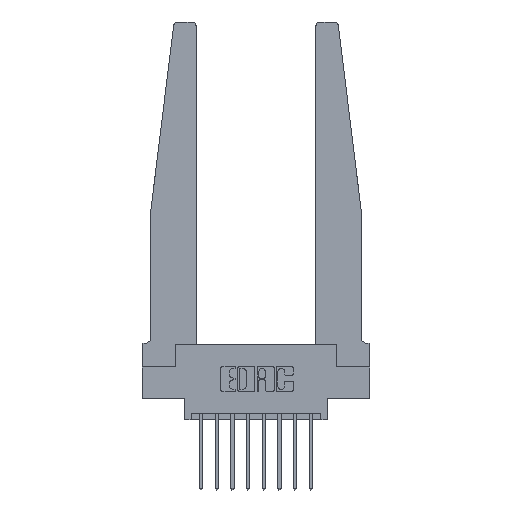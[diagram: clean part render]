
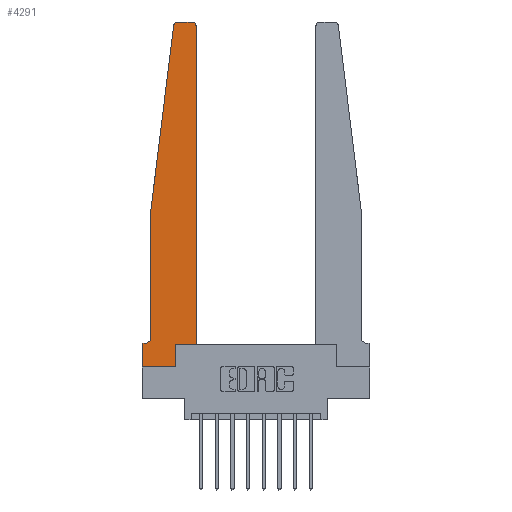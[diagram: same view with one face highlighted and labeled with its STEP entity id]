
A CAD part, top view. The second image highlights one B-rep face of the part: STEP entity #4291.
In plain terms, the highlighted planar face has unit normal (0, 0, 1).
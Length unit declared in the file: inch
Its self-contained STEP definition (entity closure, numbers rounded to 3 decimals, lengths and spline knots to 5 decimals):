
#67 = EDGE_CURVE ( 'NONE', #9984, #3799, #6321, .T. ) ;
#193 = VECTOR ( 'NONE', #11996, 39.37008 ) ;
#274 = EDGE_CURVE ( 'NONE', #8454, #6829, #14087, .T. ) ;
#299 = ORIENTED_EDGE ( 'NONE', *, *, #14269, .T. ) ;
#716 = EDGE_CURVE ( 'NONE', #3799, #8982, #1531, .T. ) ;
#754 = ORIENTED_EDGE ( 'NONE', *, *, #9614, .T. ) ;
#1057 = DIRECTION ( 'NONE',  ( -1., 0., 0. ) ) ;
#1059 = EDGE_CURVE ( 'NONE', #12440, #3065, #4650, .T. ) ;
#1168 = EDGE_LOOP ( 'NONE', ( #9666, #7972, #2958, #1210, #299, #5373, #6129, #754, #4764, #2316, #4308, #8832 ) ) ;
#1210 = ORIENTED_EDGE ( 'NONE', *, *, #10025, .T. ) ;
#1282 = CARTESIAN_POINT ( 'NONE',  ( 0.425, 2.72, 0.37 ) ) ;
#1450 = AXIS2_PLACEMENT_3D ( 'NONE', #13123, #4935, #14279 ) ;
#1531 = LINE ( 'NONE', #2763, #193 ) ;
#1636 = CIRCLE ( 'NONE', #9684, 0.03 ) ;
#1896 = CARTESIAN_POINT ( 'NONE',  ( 0.2605, 0., 0.37 ) ) ;
#1973 = VECTOR ( 'NONE', #8669, 39.37008 ) ;
#2025 = DIRECTION ( 'NONE',  ( 1., 0., 0. ) ) ;
#2316 = ORIENTED_EDGE ( 'NONE', *, *, #67, .T. ) ;
#2404 = EDGE_CURVE ( 'NONE', #3851, #9984, #12840, .T. ) ;
#2645 = DIRECTION ( 'NONE',  ( 0., 0., 1. ) ) ;
#2763 = CARTESIAN_POINT ( 'NONE',  ( 0.425, 0.18, 0.37 ) ) ;
#2958 = ORIENTED_EDGE ( 'NONE', *, *, #274, .T. ) ;
#3015 = VERTEX_POINT ( 'NONE', #11948 ) ;
#3065 = VERTEX_POINT ( 'NONE', #9951 ) ;
#3325 = LINE ( 'NONE', #12490, #8566 ) ;
#3336 = CARTESIAN_POINT ( 'NONE',  ( 0.065, 1.25, 0.37 ) ) ;
#3615 = VECTOR ( 'NONE', #6893, 39.37008 ) ;
#3698 = CARTESIAN_POINT ( 'NONE',  ( 0.24675, 2.72367, 0.37 ) ) ;
#3736 = DIRECTION ( 'NONE',  ( 1., 0., 0. ) ) ;
#3799 = VERTEX_POINT ( 'NONE', #9691 ) ;
#3851 = VERTEX_POINT ( 'NONE', #1896 ) ;
#4054 = VERTEX_POINT ( 'NONE', #12898 ) ;
#4291 = ADVANCED_FACE ( 'NONE', ( #8633 ), #8559, .T. ) ;
#4308 = ORIENTED_EDGE ( 'NONE', *, *, #716, .T. ) ;
#4323 = EDGE_CURVE ( 'NONE', #9707, #8454, #7304, .T. ) ;
#4433 = CARTESIAN_POINT ( 'NONE',  ( 0.2605, 0.18, 0.37 ) ) ;
#4650 = LINE ( 'NONE', #12597, #5790 ) ;
#4764 = ORIENTED_EDGE ( 'NONE', *, *, #2404, .T. ) ;
#4787 = DIRECTION ( 'NONE',  ( 0., 0., 1. ) ) ;
#4863 = CARTESIAN_POINT ( 'NONE',  ( 0.27653, 2.72, 0.37 ) ) ;
#4935 = DIRECTION ( 'NONE',  ( 0., 0., 1. ) ) ;
#5079 = VECTOR ( 'NONE', #5450, 39.37008 ) ;
#5373 = ORIENTED_EDGE ( 'NONE', *, *, #1059, .T. ) ;
#5410 = VECTOR ( 'NONE', #13790, 39.37008 ) ;
#5450 = DIRECTION ( 'NONE',  ( 1., 0., 0. ) ) ;
#5603 = CARTESIAN_POINT ( 'NONE',  ( 0., 0., 0.37 ) ) ;
#5790 = VECTOR ( 'NONE', #1057, 39.37008 ) ;
#6129 = ORIENTED_EDGE ( 'NONE', *, *, #12045, .T. ) ;
#6289 = LINE ( 'NONE', #10939, #1973 ) ;
#6321 = LINE ( 'NONE', #6590, #5079 ) ;
#6498 = CARTESIAN_POINT ( 'NONE',  ( 0.015, 0.1875, 0.37 ) ) ;
#6590 = CARTESIAN_POINT ( 'NONE',  ( 0.425, 0.18, 0.37 ) ) ;
#6829 = VERTEX_POINT ( 'NONE', #3336 ) ;
#6854 = VERTEX_POINT ( 'NONE', #10277 ) ;
#6893 = DIRECTION ( 'NONE',  ( -0.122, -0.992, 0. ) ) ;
#7304 = CIRCLE ( 'NONE', #13911, 0.03 ) ;
#7516 = CARTESIAN_POINT ( 'NONE',  ( 0.395, 2.72, 0.37 ) ) ;
#7972 = ORIENTED_EDGE ( 'NONE', *, *, #4323, .T. ) ;
#8387 = EDGE_CURVE ( 'NONE', #3015, #9707, #11324, .T. ) ;
#8454 = VERTEX_POINT ( 'NONE', #3698 ) ;
#8559 = PLANE ( 'NONE',  #1450 ) ;
#8566 = VECTOR ( 'NONE', #2025, 39.37008 ) ;
#8633 = FACE_OUTER_BOUND ( 'NONE', #1168, .T. ) ;
#8669 = DIRECTION ( 'NONE',  ( 0., -1., 0. ) ) ;
#8731 = AXIS2_PLACEMENT_3D ( 'NONE', #12185, #13333, #9814 ) ;
#8750 = DIRECTION ( 'NONE',  ( 1., 0., 0. ) ) ;
#8832 = ORIENTED_EDGE ( 'NONE', *, *, #14321, .T. ) ;
#8982 = VERTEX_POINT ( 'NONE', #1282 ) ;
#9127 = CARTESIAN_POINT ( 'NONE',  ( 0.065, 1.25, 0.37 ) ) ;
#9614 = EDGE_CURVE ( 'NONE', #6854, #3851, #3325, .T. ) ;
#9666 = ORIENTED_EDGE ( 'NONE', *, *, #8387, .T. ) ;
#9684 = AXIS2_PLACEMENT_3D ( 'NONE', #7516, #2645, #8750 ) ;
#9691 = CARTESIAN_POINT ( 'NONE',  ( 0.425, 0.18, 0.37 ) ) ;
#9707 = VERTEX_POINT ( 'NONE', #14954 ) ;
#9814 = DIRECTION ( 'NONE',  ( -1., 0., 0. ) ) ;
#9951 = CARTESIAN_POINT ( 'NONE',  ( 0., 0.1875, 0.37 ) ) ;
#9984 = VERTEX_POINT ( 'NONE', #12094 ) ;
#10025 = EDGE_CURVE ( 'NONE', #6829, #4054, #6289, .T. ) ;
#10277 = CARTESIAN_POINT ( 'NONE',  ( 0., 0., 0.37 ) ) ;
#10408 = LINE ( 'NONE', #5603, #5410 ) ;
#10939 = CARTESIAN_POINT ( 'NONE',  ( 0.065, 1.25, 0.37 ) ) ;
#11324 = LINE ( 'NONE', #11482, #14663 ) ;
#11482 = CARTESIAN_POINT ( 'NONE',  ( 0.25, 2.75, 0.37 ) ) ;
#11680 = DIRECTION ( 'NONE',  ( 0., 1., 0. ) ) ;
#11948 = CARTESIAN_POINT ( 'NONE',  ( 0.395, 2.75, 0.37 ) ) ;
#11996 = DIRECTION ( 'NONE',  ( 0., 1., 0. ) ) ;
#12045 = EDGE_CURVE ( 'NONE', #3065, #6854, #10408, .T. ) ;
#12094 = CARTESIAN_POINT ( 'NONE',  ( 0.2605, 0.18, 0.37 ) ) ;
#12185 = CARTESIAN_POINT ( 'NONE',  ( 0.015, 0.2375, 0.37 ) ) ;
#12440 = VERTEX_POINT ( 'NONE', #6498 ) ;
#12490 = CARTESIAN_POINT ( 'NONE',  ( 0., 0., 0.37 ) ) ;
#12597 = CARTESIAN_POINT ( 'NONE',  ( 0.065, 0.1875, 0.37 ) ) ;
#12840 = LINE ( 'NONE', #4433, #13287 ) ;
#12898 = CARTESIAN_POINT ( 'NONE',  ( 0.065, 0.2375, 0.37 ) ) ;
#13123 = CARTESIAN_POINT ( 'NONE',  ( 0., 0.1875, 0.37 ) ) ;
#13287 = VECTOR ( 'NONE', #11680, 39.37008 ) ;
#13333 = DIRECTION ( 'NONE',  ( 0., 0., -1. ) ) ;
#13790 = DIRECTION ( 'NONE',  ( 0., -1., 0. ) ) ;
#13857 = CIRCLE ( 'NONE', #8731, 0.05 ) ;
#13911 = AXIS2_PLACEMENT_3D ( 'NONE', #4863, #4787, #3736 ) ;
#14087 = LINE ( 'NONE', #9127, #3615 ) ;
#14269 = EDGE_CURVE ( 'NONE', #4054, #12440, #13857, .T. ) ;
#14279 = DIRECTION ( 'NONE',  ( 1., 0., 0. ) ) ;
#14321 = EDGE_CURVE ( 'NONE', #8982, #3015, #1636, .T. ) ;
#14663 = VECTOR ( 'NONE', #14950, 39.37008 ) ;
#14950 = DIRECTION ( 'NONE',  ( -1., 0., 0. ) ) ;
#14954 = CARTESIAN_POINT ( 'NONE',  ( 0.27653, 2.75, 0.37 ) ) ;
